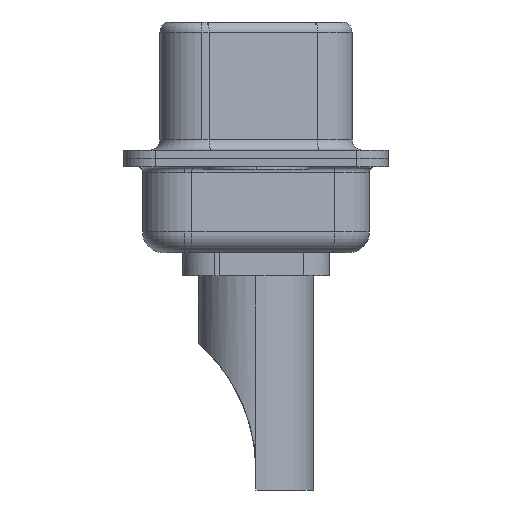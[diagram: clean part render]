
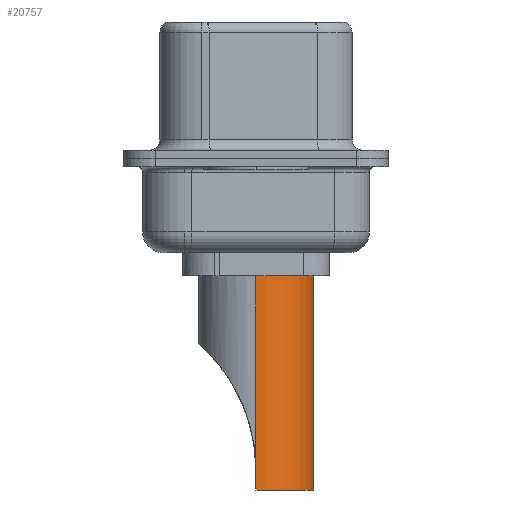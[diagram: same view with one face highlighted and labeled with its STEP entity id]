
A CAD part, left-side view. The second image highlights one B-rep face of the part: STEP entity #20757.
In plain terms, the highlighted cylindrical face has radius 2.75 mm (diameter 5.5 mm), a partial arc.
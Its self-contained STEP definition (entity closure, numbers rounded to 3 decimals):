
#167 = VERTEX_POINT ( 'NONE', #10758 ) ;
#514 = VECTOR ( 'NONE', #5624, 1000. ) ;
#1066 = CARTESIAN_POINT ( 'NONE',  ( -2.75, 0., -7.764 ) ) ;
#1185 = CIRCLE ( 'NONE', #10462, 2.75 ) ;
#1913 = CARTESIAN_POINT ( 'NONE',  ( -2.75, 0., 4.234 ) ) ;
#2018 = AXIS2_PLACEMENT_3D ( 'NONE', #9345, #4181, #7653 ) ;
#2332 = DIRECTION ( 'NONE',  ( 0., 0., 1. ) ) ;
#2398 = EDGE_CURVE ( 'NONE', #15927, #17329, #1185, .T. ) ;
#2688 = ORIENTED_EDGE ( 'NONE', *, *, #17396, .T. ) ;
#2719 = CARTESIAN_POINT ( 'NONE',  ( 2.75, 0., -7.764 ) ) ;
#3136 = CARTESIAN_POINT ( 'NONE',  ( 0., 0., 1.5 ) ) ;
#3241 = EDGE_CURVE ( 'NONE', #6702, #5906, #19515, .T. ) ;
#4181 = DIRECTION ( 'NONE',  ( 0., 0., 1. ) ) ;
#4807 = DIRECTION ( 'NONE',  ( 1., 0., 0. ) ) ;
#5522 = CARTESIAN_POINT ( 'NONE',  ( 0., 0., -8.7 ) ) ;
#5624 = DIRECTION ( 'NONE',  ( 0., 0., -1. ) ) ;
#5852 = DIRECTION ( 'NONE',  ( 0., 0., -1. ) ) ;
#5906 = VERTEX_POINT ( 'NONE', #9905 ) ;
#6397 = ORIENTED_EDGE ( 'NONE', *, *, #3241, .F. ) ;
#6532 = ORIENTED_EDGE ( 'NONE', *, *, #2398, .T. ) ;
#6702 = VERTEX_POINT ( 'NONE', #1066 ) ;
#7333 = CARTESIAN_POINT ( 'NONE',  ( 2.75, 0., -8.7 ) ) ;
#7653 = DIRECTION ( 'NONE',  ( 1., 0., 0. ) ) ;
#9345 = CARTESIAN_POINT ( 'NONE',  ( 0., 0., 4.234 ) ) ;
#9905 = CARTESIAN_POINT ( 'NONE',  ( -2.75, 0., 1.5 ) ) ;
#10377 = DIRECTION ( 'NONE',  ( 0., 0., 1. ) ) ;
#10462 = AXIS2_PLACEMENT_3D ( 'NONE', #5522, #20041, #21363 ) ;
#10758 = CARTESIAN_POINT ( 'NONE',  ( 2.75, 0., 1.5 ) ) ;
#11408 = ORIENTED_EDGE ( 'NONE', *, *, #16697, .T. ) ;
#11633 = VECTOR ( 'NONE', #5852, 1000. ) ;
#11921 = VECTOR ( 'NONE', #2332, 1000. ) ;
#12451 = ORIENTED_EDGE ( 'NONE', *, *, #16989, .F. ) ;
#12507 = EDGE_CURVE ( 'NONE', #16852, #17329, #13954, .T. ) ;
#12908 = AXIS2_PLACEMENT_3D ( 'NONE', #3136, #14857, #4807 ) ;
#13824 = ORIENTED_EDGE ( 'NONE', *, *, #12507, .F. ) ;
#13954 = LINE ( 'NONE', #7333, #514 ) ;
#14066 = CARTESIAN_POINT ( 'NONE',  ( 2.75, 0., -8.7 ) ) ;
#14857 = DIRECTION ( 'NONE',  ( 0., 0., 1. ) ) ;
#15927 = VERTEX_POINT ( 'NONE', #18829 ) ;
#16697 = EDGE_CURVE ( 'NONE', #16852, #167, #20770, .T. ) ;
#16852 = VERTEX_POINT ( 'NONE', #2719 ) ;
#16989 = EDGE_CURVE ( 'NONE', #5906, #167, #19996, .T. ) ;
#17329 = VERTEX_POINT ( 'NONE', #14066 ) ;
#17396 = EDGE_CURVE ( 'NONE', #6702, #15927, #20486, .T. ) ;
#17590 = CARTESIAN_POINT ( 'NONE',  ( -2.75, 0., -8.7 ) ) ;
#17997 = EDGE_LOOP ( 'NONE', ( #6397, #2688, #6532, #13824, #11408, #12451 ) ) ;
#18829 = CARTESIAN_POINT ( 'NONE',  ( -2.75, 0., -8.7 ) ) ;
#18989 = VECTOR ( 'NONE', #10377, 1000. ) ;
#19515 = LINE ( 'NONE', #1913, #18989 ) ;
#19996 = CIRCLE ( 'NONE', #12908, 2.75 ) ;
#20041 = DIRECTION ( 'NONE',  ( 0., 0., 1. ) ) ;
#20486 = LINE ( 'NONE', #17590, #11633 ) ;
#20670 = CARTESIAN_POINT ( 'NONE',  ( 2.75, 0., 4.234 ) ) ;
#20757 = ADVANCED_FACE ( 'NONE', ( #21687 ), #21157, .T. ) ;
#20770 = LINE ( 'NONE', #20670, #11921 ) ;
#21157 = CYLINDRICAL_SURFACE ( 'NONE', #2018, 2.75 ) ;
#21363 = DIRECTION ( 'NONE',  ( 1., 0., 0. ) ) ;
#21687 = FACE_OUTER_BOUND ( 'NONE', #17997, .T. ) ;
